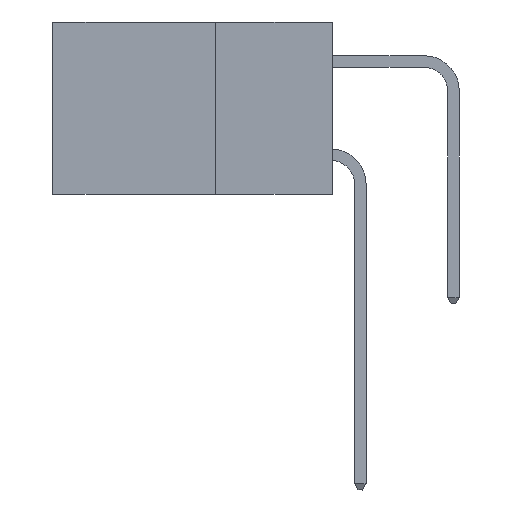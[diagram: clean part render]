
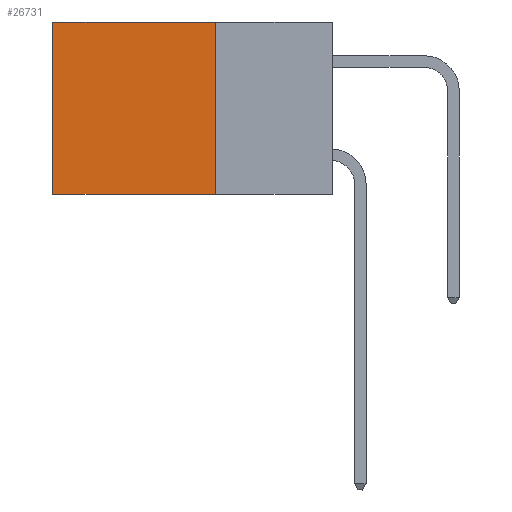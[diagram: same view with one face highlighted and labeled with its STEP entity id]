
A CAD part, left-side view. The second image highlights one B-rep face of the part: STEP entity #26731.
In plain terms, the highlighted planar face has unit normal (-1, 0, 0).
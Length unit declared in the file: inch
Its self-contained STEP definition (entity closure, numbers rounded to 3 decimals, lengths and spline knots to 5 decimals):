
#1280 = CARTESIAN_POINT ( 'NONE',  ( 0.2615, 0.25, -0.37 ) ) ;
#1505 = CARTESIAN_POINT ( 'NONE',  ( 0.2615, 0.25, 0. ) ) ;
#1874 = DIRECTION ( 'NONE',  ( 1., 0., 0. ) ) ;
#2178 = LINE ( 'NONE', #24828, #23872 ) ;
#3244 = EDGE_CURVE ( 'NONE', #26867, #6399, #20859, .T. ) ;
#3725 = ORIENTED_EDGE ( 'NONE', *, *, #15328, .F. ) ;
#4289 = AXIS2_PLACEMENT_3D ( 'NONE', #8545, #1874, #6504 ) ;
#6238 = PLANE ( 'NONE',  #4289 ) ;
#6399 = VERTEX_POINT ( 'NONE', #1280 ) ;
#6504 = DIRECTION ( 'NONE',  ( 0., 0., -1. ) ) ;
#8545 = CARTESIAN_POINT ( 'NONE',  ( 0.2615, 0.25, -0.37 ) ) ;
#8626 = VECTOR ( 'NONE', #25943, 39.37008 ) ;
#8786 = ORIENTED_EDGE ( 'NONE', *, *, #20935, .T. ) ;
#9683 = ORIENTED_EDGE ( 'NONE', *, *, #3244, .F. ) ;
#10061 = CARTESIAN_POINT ( 'NONE',  ( 0.2615, 0.25, -0.37 ) ) ;
#10228 = VECTOR ( 'NONE', #10335, 39.37008 ) ;
#10335 = DIRECTION ( 'NONE',  ( 0., 1., 0. ) ) ;
#10645 = VERTEX_POINT ( 'NONE', #10773 ) ;
#10773 = CARTESIAN_POINT ( 'NONE',  ( 0.2615, 0.6, -0.37 ) ) ;
#10852 = EDGE_LOOP ( 'NONE', ( #8786, #3725, #9683, #24127 ) ) ;
#12104 = CARTESIAN_POINT ( 'NONE',  ( 0.2615, 0.25, -0.37 ) ) ;
#12405 = CARTESIAN_POINT ( 'NONE',  ( 0.2615, 0.6, 0. ) ) ;
#12500 = VERTEX_POINT ( 'NONE', #12405 ) ;
#13908 = LINE ( 'NONE', #1505, #8626 ) ;
#14527 = FACE_OUTER_BOUND ( 'NONE', #10852, .T. ) ;
#15328 = EDGE_CURVE ( 'NONE', #6399, #10645, #22775, .T. ) ;
#20488 = DIRECTION ( 'NONE',  ( 0., 0., -1. ) ) ;
#20821 = EDGE_CURVE ( 'NONE', #26867, #12500, #13908, .T. ) ;
#20859 = LINE ( 'NONE', #12104, #21396 ) ;
#20935 = EDGE_CURVE ( 'NONE', #12500, #10645, #2178, .T. ) ;
#21396 = VECTOR ( 'NONE', #25193, 39.37008 ) ;
#22775 = LINE ( 'NONE', #10061, #10228 ) ;
#23408 = CARTESIAN_POINT ( 'NONE',  ( 0.2615, 0.25, 0. ) ) ;
#23872 = VECTOR ( 'NONE', #20488, 39.37008 ) ;
#24127 = ORIENTED_EDGE ( 'NONE', *, *, #20821, .T. ) ;
#24828 = CARTESIAN_POINT ( 'NONE',  ( 0.2615, 0.6, -0.37 ) ) ;
#25193 = DIRECTION ( 'NONE',  ( 0., 0., -1. ) ) ;
#25943 = DIRECTION ( 'NONE',  ( 0., 1., 0. ) ) ;
#26731 = ADVANCED_FACE ( 'NONE', ( #14527 ), #6238, .F. ) ;
#26867 = VERTEX_POINT ( 'NONE', #23408 ) ;
